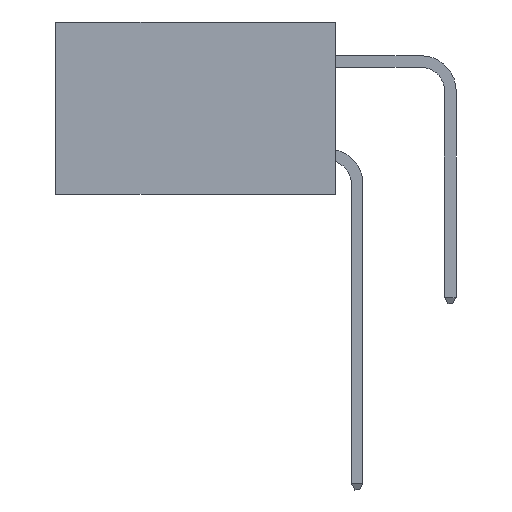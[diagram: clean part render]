
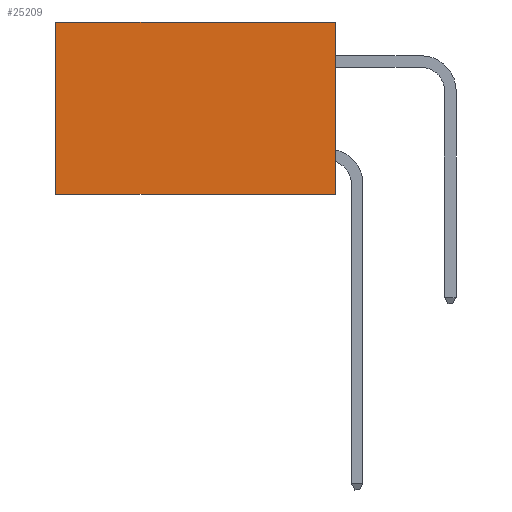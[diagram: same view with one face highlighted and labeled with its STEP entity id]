
A CAD part, left-side view. The second image highlights one B-rep face of the part: STEP entity #25209.
In plain terms, the highlighted planar face has unit normal (-1, 0, 0).
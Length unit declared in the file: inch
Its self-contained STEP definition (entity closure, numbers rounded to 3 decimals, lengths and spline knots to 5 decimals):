
#66 = PLANE ( 'NONE',  #20824 ) ;
#646 = CARTESIAN_POINT ( 'NONE',  ( 0.2875, 0., 0. ) ) ;
#1004 = DIRECTION ( 'NONE',  ( 0., 0., -1. ) ) ;
#3087 = LINE ( 'NONE', #646, #4752 ) ;
#4091 = DIRECTION ( 'NONE',  ( 0., 1., 0. ) ) ;
#4752 = VECTOR ( 'NONE', #31939, 39.37008 ) ;
#4929 = VECTOR ( 'NONE', #14636, 39.37008 ) ;
#5047 = CARTESIAN_POINT ( 'NONE',  ( 0.2875, 0.6, 0. ) ) ;
#5198 = DIRECTION ( 'NONE',  ( 0., 0., -1. ) ) ;
#8287 = CARTESIAN_POINT ( 'NONE',  ( 0.2875, 0., -0.37 ) ) ;
#9672 = VERTEX_POINT ( 'NONE', #31207 ) ;
#10643 = ORIENTED_EDGE ( 'NONE', *, *, #13495, .F. ) ;
#12202 = EDGE_CURVE ( 'NONE', #17894, #9672, #28906, .T. ) ;
#12977 = ORIENTED_EDGE ( 'NONE', *, *, #12202, .F. ) ;
#13495 = EDGE_CURVE ( 'NONE', #26429, #17894, #28480, .T. ) ;
#14636 = DIRECTION ( 'NONE',  ( 0., 0., -1. ) ) ;
#15990 = EDGE_CURVE ( 'NONE', #26429, #21386, #3087, .T. ) ;
#16194 = CARTESIAN_POINT ( 'NONE',  ( 0.2875, 0., 0. ) ) ;
#17894 = VERTEX_POINT ( 'NONE', #8287 ) ;
#19010 = VECTOR ( 'NONE', #1004, 39.37008 ) ;
#19120 = ORIENTED_EDGE ( 'NONE', *, *, #19601, .T. ) ;
#19601 = EDGE_CURVE ( 'NONE', #21386, #9672, #27102, .T. ) ;
#20300 = ORIENTED_EDGE ( 'NONE', *, *, #15990, .T. ) ;
#20805 = DIRECTION ( 'NONE',  ( 1., 0., 0. ) ) ;
#20824 = AXIS2_PLACEMENT_3D ( 'NONE', #33647, #20805, #5198 ) ;
#21386 = VERTEX_POINT ( 'NONE', #5047 ) ;
#21402 = CARTESIAN_POINT ( 'NONE',  ( 0.2875, 0.6, 0. ) ) ;
#21663 = VECTOR ( 'NONE', #4091, 39.37008 ) ;
#22394 = CARTESIAN_POINT ( 'NONE',  ( 0.2875, 0., -0.37 ) ) ;
#24324 = FACE_OUTER_BOUND ( 'NONE', #32243, .T. ) ;
#25209 = ADVANCED_FACE ( 'NONE', ( #24324 ), #66, .F. ) ;
#26429 = VERTEX_POINT ( 'NONE', #16194 ) ;
#27102 = LINE ( 'NONE', #21402, #19010 ) ;
#27548 = CARTESIAN_POINT ( 'NONE',  ( 0.2875, 0., 0. ) ) ;
#28480 = LINE ( 'NONE', #27548, #4929 ) ;
#28906 = LINE ( 'NONE', #22394, #21663 ) ;
#31207 = CARTESIAN_POINT ( 'NONE',  ( 0.2875, 0.6, -0.37 ) ) ;
#31939 = DIRECTION ( 'NONE',  ( 0., 1., 0. ) ) ;
#32243 = EDGE_LOOP ( 'NONE', ( #19120, #12977, #10643, #20300 ) ) ;
#33647 = CARTESIAN_POINT ( 'NONE',  ( 0.2875, 0., 0. ) ) ;
